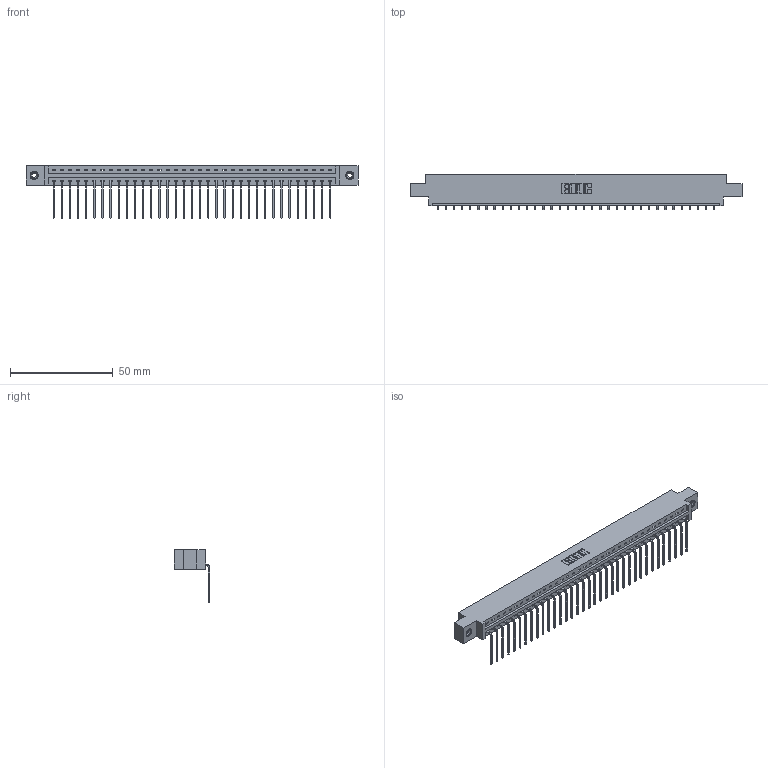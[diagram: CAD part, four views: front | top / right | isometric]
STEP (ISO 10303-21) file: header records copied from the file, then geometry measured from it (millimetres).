
FILE_DESCRIPTION (( 'STEP AP203' ), '1' );
FILE_NAME ('337-035-559-608.STEP', '2019-10-01T13:29:12', ( '' ), ( '' ), 'SwSTEP 2.0', 'SolidWorks 2016', '' );
FILE_SCHEMA (( 'CONFIG_CONTROL_DESIGN' ));
Length unit declared in the file: inch
Products named in the file (4): 337-035-559-608; 345-292-001_558 559 Tail - 1; 337 Part_0.170 Offset - 0.156 Dia-TI; 345-250-001_345-250-003-102
Assembly tree (38 placements, depth 2):
  337-035-559-608
    337 Part_0.170 Offset - 0.156 Dia-TI
    345-292-001_558 559 Tail - 1  x35
    345-250-001_345-250-003-102  x2
Bounding box: 161.7 x 17.09 x 25.53 mm (x, y, z)
Volume: 16710.6 mm3; surface area: 18071.6 mm2
Topology: 38 solids, 38 shells, 2418 faces, 7249 edges, 4778 vertices
Faces by surface type: plane 1786, cylinder 616, cone 12, torus 4
Entity records: 28324 total; most frequent: CARTESIAN_POINT 4914, ORIENTED_EDGE 4878, DIRECTION 4183, EDGE_CURVE 2439, VECTOR 2291, LINE 2291, VERTEX_POINT 1620, AXIS2_PLACEMENT_3D 946
